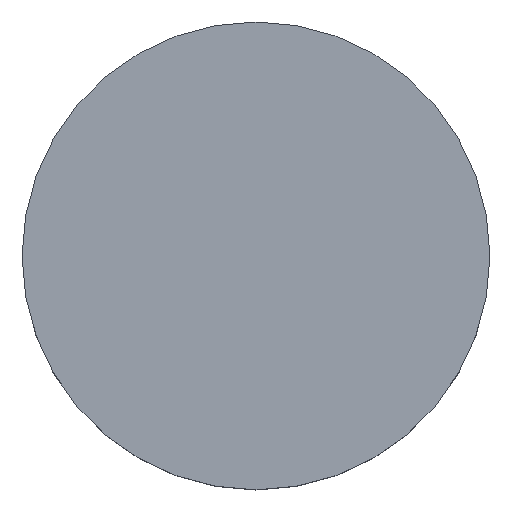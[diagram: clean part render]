
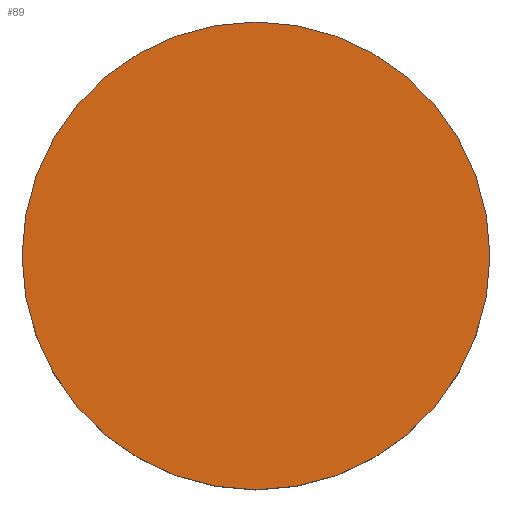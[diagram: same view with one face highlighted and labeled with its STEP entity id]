
A CAD part, top view. The second image highlights one B-rep face of the part: STEP entity #89.
In plain terms, the highlighted planar face has unit normal (0, 0, 1).
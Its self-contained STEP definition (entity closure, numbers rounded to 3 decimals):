
#25 = DIRECTION ( 'NONE',  ( 0., 0., -1. ) ) ;
#28 = DIRECTION ( 'NONE',  ( -1., 0., 0. ) ) ;
#35 = ORIENTED_EDGE ( 'NONE', *, *, #46, .T. ) ;
#37 = CARTESIAN_POINT ( 'NONE',  ( 0., 0., 1.25 ) ) ;
#42 = PLANE ( 'NONE',  #88 ) ;
#46 = EDGE_CURVE ( 'NONE', #71, #62, #53, .T. ) ;
#53 = CIRCLE ( 'NONE', #64, 5.625 ) ;
#54 = DIRECTION ( 'NONE',  ( 1., 0., 0. ) ) ;
#55 = CARTESIAN_POINT ( 'NONE',  ( 0., 0., 1.25 ) ) ;
#56 = DIRECTION ( 'NONE',  ( 0., 0., 1. ) ) ;
#62 = VERTEX_POINT ( 'NONE', #85 ) ;
#63 = CARTESIAN_POINT ( 'NONE',  ( 0., 0., 1.25 ) ) ;
#64 = AXIS2_PLACEMENT_3D ( 'NONE', #55, #56, #54 ) ;
#71 = VERTEX_POINT ( 'NONE', #79 ) ;
#79 = CARTESIAN_POINT ( 'NONE',  ( -5.625, 0., 1.25 ) ) ;
#80 = DIRECTION ( 'NONE',  ( 0., 0., 1. ) ) ;
#81 = DIRECTION ( 'NONE',  ( 1., 0., 0. ) ) ;
#85 = CARTESIAN_POINT ( 'NONE',  ( 5.625, 0., 1.25 ) ) ;
#88 = AXIS2_PLACEMENT_3D ( 'NONE', #37, #25, #28 ) ;
#89 = ADVANCED_FACE ( 'NONE', ( #113 ), #42, .F. ) ;
#92 = ORIENTED_EDGE ( 'NONE', *, *, #140, .T. ) ;
#113 = FACE_OUTER_BOUND ( 'NONE', #135, .T. ) ;
#126 = AXIS2_PLACEMENT_3D ( 'NONE', #63, #80, #81 ) ;
#134 = CIRCLE ( 'NONE', #126, 5.625 ) ;
#135 = EDGE_LOOP ( 'NONE', ( #92, #35 ) ) ;
#140 = EDGE_CURVE ( 'NONE', #62, #71, #134, .T. ) ;
